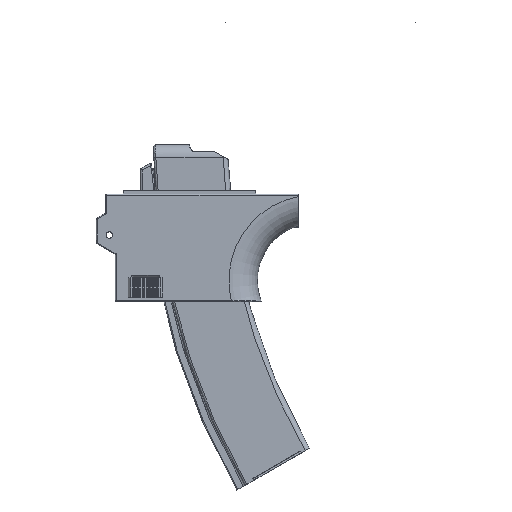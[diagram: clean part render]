
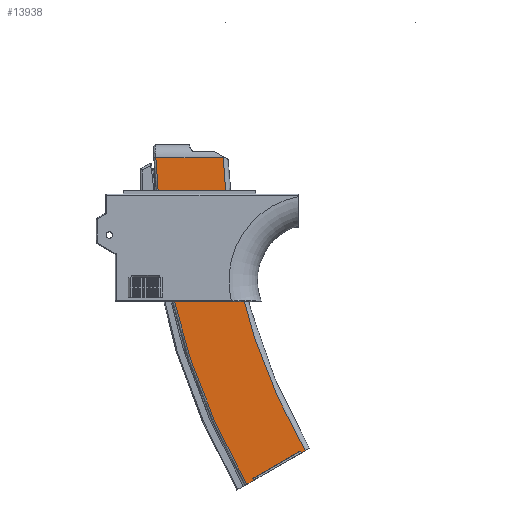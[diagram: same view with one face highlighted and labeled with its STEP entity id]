
A CAD part, top view. The second image highlights one B-rep face of the part: STEP entity #13938.
In plain terms, the highlighted planar face has unit normal (0, 0, 1).
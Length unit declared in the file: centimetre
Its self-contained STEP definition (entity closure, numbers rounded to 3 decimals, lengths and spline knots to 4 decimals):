
#514=PLANE($,#14899);
#817=CIRCLE($,#14886,35.8);
#823=CIRCLE($,#14900,32.25);
#1211=FACE_OUTER_BOUND($,#2060,.T.);
#2060=EDGE_LOOP($,(#9679,#9680,#9681,#9682,#9683,#9684,#9685,#9686));
#2914=LINE($,#19237,#3915);
#2948=LINE($,#19688,#3949);
#2958=LINE($,#19715,#3959);
#2959=LINE($,#19720,#3960);
#2960=LINE($,#19721,#3961);
#2961=LINE($,#19722,#3962);
#3915=VECTOR($,#15947,2.9);
#3949=VECTOR($,#16125,0.1);
#3959=VECTOR($,#16155,0.1);
#3960=VECTOR($,#16160,3.5508);
#3961=VECTOR($,#16161,0.398);
#3962=VECTOR($,#16162,0.252);
#5777=VERTEX_POINT($,#19234);
#5778=VERTEX_POINT($,#19236);
#5807=VERTEX_POINT($,#19504);
#5840=VERTEX_POINT($,#19682);
#5841=VERTEX_POINT($,#19687);
#5848=VERTEX_POINT($,#19713);
#5849=VERTEX_POINT($,#19717);
#5850=VERTEX_POINT($,#19718);
#7207=EDGE_CURVE($,#5778,#5777,#2914,.T.);
#7300=EDGE_CURVE($,#5840,#5807,#817,.T.);
#7302=EDGE_CURVE($,#5778,#5841,#2948,.T.);
#7316=EDGE_CURVE($,#5848,#5777,#2958,.T.);
#7317=EDGE_CURVE($,#5849,#5850,#823,.T.);
#7318=EDGE_CURVE($,#5807,#5849,#2959,.T.);
#7319=EDGE_CURVE($,#5840,#5841,#2960,.T.);
#7320=EDGE_CURVE($,#5848,#5850,#2961,.T.);
#9679=ORIENTED_EDGE($,*,*,#7317,.F.);
#9680=ORIENTED_EDGE($,*,*,#7318,.F.);
#9681=ORIENTED_EDGE($,*,*,#7300,.F.);
#9682=ORIENTED_EDGE($,*,*,#7319,.T.);
#9683=ORIENTED_EDGE($,*,*,#7302,.F.);
#9684=ORIENTED_EDGE($,*,*,#7207,.T.);
#9685=ORIENTED_EDGE($,*,*,#7316,.F.);
#9686=ORIENTED_EDGE($,*,*,#7320,.T.);
#13938=ADVANCED_FACE($,(#1211),#514,.F.);
#14886=AXIS2_PLACEMENT_3D($,#19684,#16119,#16120);
#14899=AXIS2_PLACEMENT_3D($,#19716,#16156,#16157);
#14900=AXIS2_PLACEMENT_3D($,#19719,#16158,#16159);
#15947=DIRECTION($,(0.866,0.5,0.));
#16119=DIRECTION('center_axis',(0.,0.,
-1.));
#16120=DIRECTION('ref_axis',(-0.963,-0.268,0.));
#16125=DIRECTION($,(0.5,-0.866,0.));
#16155=DIRECTION($,(-0.5,0.866,0.));
#16156=DIRECTION('center_axis',(0.,0.,
-1.));
#16157=DIRECTION('ref_axis',(0.866,0.5,0.));
#16158=DIRECTION('center_axis',(0.,0.,
1.));
#16159=DIRECTION('ref_axis',(-0.96,-0.279,0.));
#16160=DIRECTION($,(1.,0.,0.));
#16161=DIRECTION($,(0.866,0.5,0.));
#16162=DIRECTION($,(0.866,0.5,0.));
#19234=CARTESIAN_POINT('',(1.2504,-14.3698,1.1563));
#19236=CARTESIAN_POINT('',(-1.2611,-15.8198,1.1563));
#19237=CARTESIAN_POINT($,(14.6097,-6.6568,1.1563));
#19504=CARTESIAN_POINT('',(-6.3452,1.0946,1.1563));
#19682=CARTESIAN_POINT('',(-1.5558,-16.1054,1.1563));
#19684=CARTESIAN_POINT('Origin',(29.4479,1.7946,1.1563));
#19687=CARTESIAN_POINT('',(-1.2111,-15.9064,1.1563));
#19688=CARTESIAN_POINT($,(-0.9611,-16.3394,1.1563));
#19713=CARTESIAN_POINT('',(1.3004,-14.4564,1.1563));
#19715=CARTESIAN_POINT($,(1.5504,-14.8894,1.1563));
#19716=CARTESIAN_POINT('Origin',(29.4479,1.7946,1.1563));
#19717=CARTESIAN_POINT('',(-2.7945,1.0946,1.1563));
#19718=CARTESIAN_POINT('',(1.5186,-14.3304,1.1563));
#19719=CARTESIAN_POINT('Origin',(29.4479,1.7946,1.1563));
#19720=CARTESIAN_POINT($,(28.9479,1.0946,1.1563));
#19721=CARTESIAN_POINT($,(29.881,2.0446,1.1563));
#19722=CARTESIAN_POINT($,(29.881,2.0446,1.1563));
